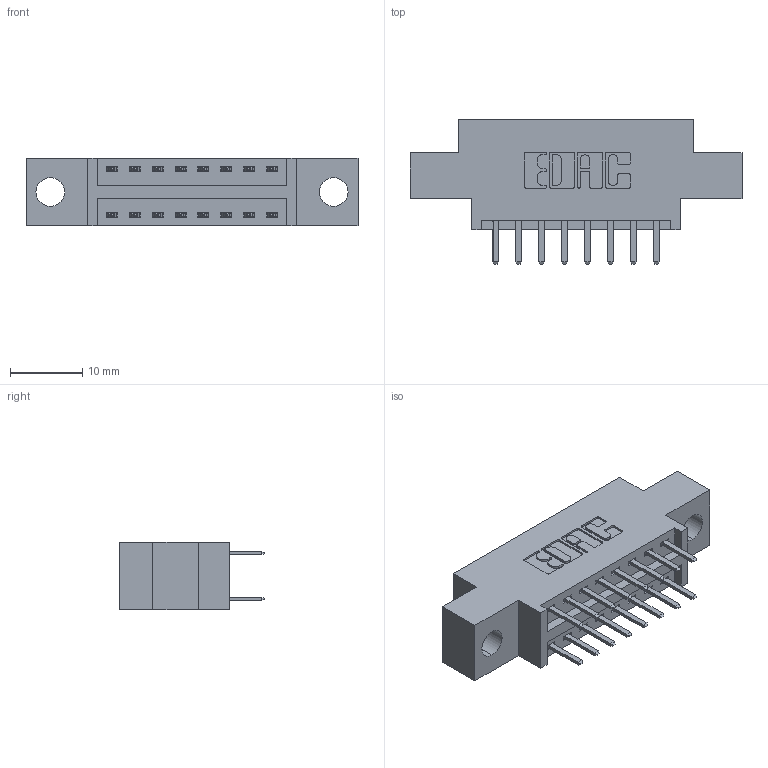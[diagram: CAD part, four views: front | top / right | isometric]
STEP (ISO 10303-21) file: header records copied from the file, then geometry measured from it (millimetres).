
FILE_DESCRIPTION (( 'STEP AP203' ), '1' );
FILE_NAME ('346-016-520-804.STEP', '2022-05-18T15:24:04', ( '' ), ( '' ), 'SwSTEP 2.0', 'SolidWorks 2020', '' );
FILE_SCHEMA (( 'CONFIG_CONTROL_DESIGN' ));
Length unit declared in the file: inch
Products named in the file (3): 346 Part_0.170 Offset - 0.156 Dia-TH; 345-292-001_345-293-120; 346-016-520-804
Assembly tree (17 placements, depth 2):
  346-016-520-804
    346 Part_0.170 Offset - 0.156 Dia-TH
    345-292-001_345-293-120  x16
Bounding box: 45.97 x 20.02 x 9.4 mm (x, y, z)
Volume: 3951.4 mm3; surface area: 4908.1 mm2
Topology: 17 solids, 17 shells, 1036 faces, 2985 edges, 1946 vertices
Faces by surface type: plane 686, cylinder 350
Entity records: 10463 total; most frequent: CARTESIAN_POINT 1790, ORIENTED_EDGE 1710, DIRECTION 1615, EDGE_CURVE 855, LINE 687, VECTOR 687, VERTEX_POINT 566, AXIS2_PLACEMENT_3D 464
